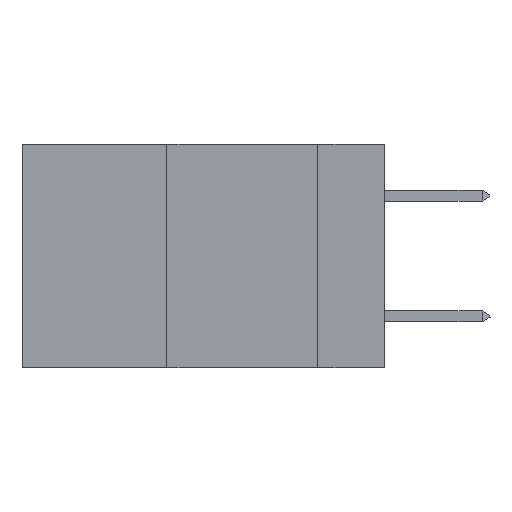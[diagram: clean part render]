
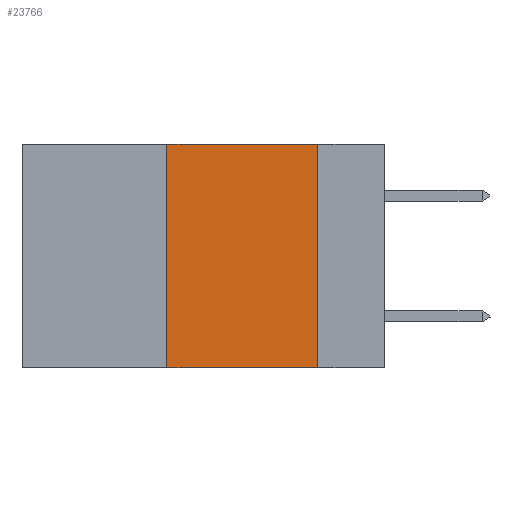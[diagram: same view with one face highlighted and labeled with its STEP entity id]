
A CAD part, left-side view. The second image highlights one B-rep face of the part: STEP entity #23766.
In plain terms, the highlighted planar face has unit normal (-1, 0, 0).
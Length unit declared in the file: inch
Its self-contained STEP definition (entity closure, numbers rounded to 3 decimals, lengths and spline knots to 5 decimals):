
#415 = LINE ( 'NONE', #12972, #22248 ) ;
#742 = AXIS2_PLACEMENT_3D ( 'NONE', #17747, #1101, #11774 ) ;
#793 = ORIENTED_EDGE ( 'NONE', *, *, #19690, .T. ) ;
#909 = EDGE_CURVE ( 'NONE', #9738, #26698, #15463, .T. ) ;
#1101 = DIRECTION ( 'NONE',  ( 1., 0., 0. ) ) ;
#3981 = DIRECTION ( 'NONE',  ( 0., -1., 0. ) ) ;
#4572 = VECTOR ( 'NONE', #3981, 39.37008 ) ;
#6125 = DIRECTION ( 'NONE',  ( 0., 0., 1. ) ) ;
#6440 = CARTESIAN_POINT ( 'NONE',  ( 0., 0.11, 0. ) ) ;
#7620 = VECTOR ( 'NONE', #22265, 39.37008 ) ;
#8008 = ORIENTED_EDGE ( 'NONE', *, *, #12051, .F. ) ;
#9738 = VERTEX_POINT ( 'NONE', #17689 ) ;
#9896 = CARTESIAN_POINT ( 'NONE',  ( 0., 0.6, 0. ) ) ;
#10189 = CARTESIAN_POINT ( 'NONE',  ( 0., 0.36, 0. ) ) ;
#11699 = ORIENTED_EDGE ( 'NONE', *, *, #13605, .F. ) ;
#11774 = DIRECTION ( 'NONE',  ( 0., 0., -1. ) ) ;
#12051 = EDGE_CURVE ( 'NONE', #26698, #17828, #415, .T. ) ;
#12972 = CARTESIAN_POINT ( 'NONE',  ( 0., 0.11, 0. ) ) ;
#13605 = EDGE_CURVE ( 'NONE', #17043, #9738, #23171, .T. ) ;
#15463 = LINE ( 'NONE', #9896, #4572 ) ;
#16437 = FACE_OUTER_BOUND ( 'NONE', #19402, .T. ) ;
#17043 = VERTEX_POINT ( 'NONE', #18939 ) ;
#17689 = CARTESIAN_POINT ( 'NONE',  ( 0., 0.36, 0. ) ) ;
#17747 = CARTESIAN_POINT ( 'NONE',  ( 0., 0.6, 0. ) ) ;
#17828 = VERTEX_POINT ( 'NONE', #22305 ) ;
#18939 = CARTESIAN_POINT ( 'NONE',  ( 0., 0.36, -0.37 ) ) ;
#19142 = ORIENTED_EDGE ( 'NONE', *, *, #909, .F. ) ;
#19402 = EDGE_LOOP ( 'NONE', ( #8008, #19142, #11699, #793 ) ) ;
#19690 = EDGE_CURVE ( 'NONE', #17043, #17828, #20115, .T. ) ;
#20115 = LINE ( 'NONE', #24412, #7620 ) ;
#21421 = DIRECTION ( 'NONE',  ( 0., 0., -1. ) ) ;
#22248 = VECTOR ( 'NONE', #21421, 39.37008 ) ;
#22265 = DIRECTION ( 'NONE',  ( 0., -1., 0. ) ) ;
#22305 = CARTESIAN_POINT ( 'NONE',  ( 0., 0.11, -0.37 ) ) ;
#23171 = LINE ( 'NONE', #10189, #26821 ) ;
#23766 = ADVANCED_FACE ( 'NONE', ( #16437 ), #24296, .F. ) ;
#24296 = PLANE ( 'NONE',  #742 ) ;
#24412 = CARTESIAN_POINT ( 'NONE',  ( 0., 0.6, -0.37 ) ) ;
#26698 = VERTEX_POINT ( 'NONE', #6440 ) ;
#26821 = VECTOR ( 'NONE', #6125, 39.37008 ) ;
